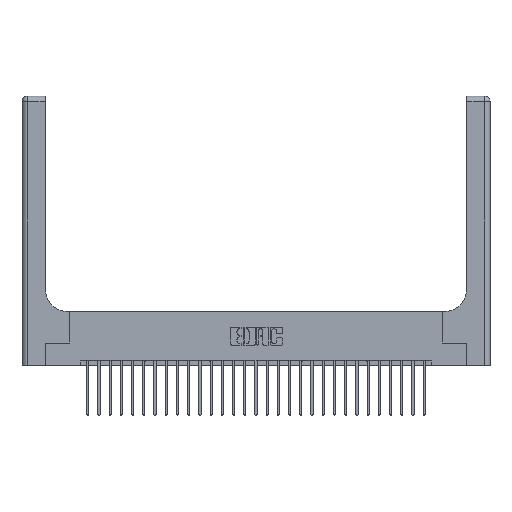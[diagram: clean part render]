
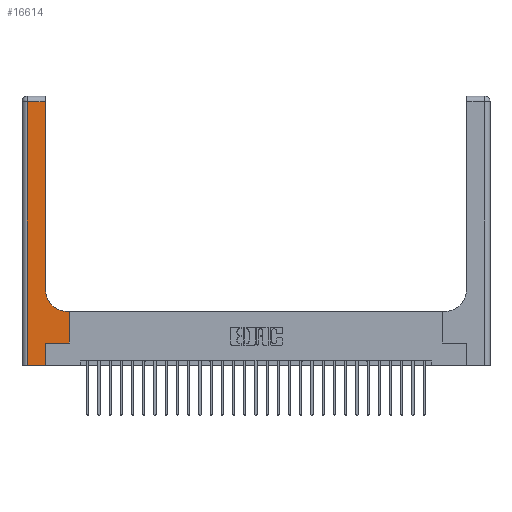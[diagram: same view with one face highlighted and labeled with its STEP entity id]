
A CAD part, top view. The second image highlights one B-rep face of the part: STEP entity #16614.
In plain terms, the highlighted planar face has unit normal (0, 0, 1).
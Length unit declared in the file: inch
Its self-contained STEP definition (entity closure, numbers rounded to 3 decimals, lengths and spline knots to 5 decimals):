
#971 = VERTEX_POINT ( 'NONE', #20135 ) ;
#1554 = DIRECTION ( 'NONE',  ( 0., 0., -1. ) ) ;
#1675 = CARTESIAN_POINT ( 'NONE',  ( 0.06, 0., 0.37 ) ) ;
#1755 = EDGE_CURVE ( 'NONE', #26355, #6353, #17251, .T. ) ;
#1874 = AXIS2_PLACEMENT_3D ( 'NONE', #26475, #1554, #7898 ) ;
#1891 = CARTESIAN_POINT ( 'NONE',  ( 0., 2.94, 0.37 ) ) ;
#2006 = AXIS2_PLACEMENT_3D ( 'NONE', #8430, #20499, #18570 ) ;
#2599 = VERTEX_POINT ( 'NONE', #3505 ) ;
#3308 = VECTOR ( 'NONE', #17036, 39.37008 ) ;
#3505 = CARTESIAN_POINT ( 'NONE',  ( 0.26, 2.94, 0.37 ) ) ;
#4293 = EDGE_CURVE ( 'NONE', #17906, #971, #13842, .T. ) ;
#4550 = CARTESIAN_POINT ( 'NONE',  ( 0.06, 2.94, 0.37 ) ) ;
#6353 = VERTEX_POINT ( 'NONE', #23645 ) ;
#7100 = LINE ( 'NONE', #15888, #16823 ) ;
#7628 = VERTEX_POINT ( 'NONE', #26012 ) ;
#7898 = DIRECTION ( 'NONE',  ( 1., 0., 0. ) ) ;
#8225 = DIRECTION ( 'NONE',  ( -1., 0., 0. ) ) ;
#8430 = CARTESIAN_POINT ( 'NONE',  ( 0., 3., 0.37 ) ) ;
#8504 = ORIENTED_EDGE ( 'NONE', *, *, #1755, .T. ) ;
#9258 = LINE ( 'NONE', #1891, #19678 ) ;
#9851 = CARTESIAN_POINT ( 'NONE',  ( 0.528, 0.25, 0.37 ) ) ;
#10136 = LINE ( 'NONE', #21403, #3308 ) ;
#10142 = ORIENTED_EDGE ( 'NONE', *, *, #13453, .T. ) ;
#11033 = ORIENTED_EDGE ( 'NONE', *, *, #4293, .T. ) ;
#11135 = CARTESIAN_POINT ( 'NONE',  ( 0.528, 0.25, 0.37 ) ) ;
#11795 = ORIENTED_EDGE ( 'NONE', *, *, #24384, .T. ) ;
#12333 = DIRECTION ( 'NONE',  ( 0., -1., 0. ) ) ;
#12612 = EDGE_CURVE ( 'NONE', #7628, #24047, #19291, .T. ) ;
#13453 = EDGE_CURVE ( 'NONE', #6353, #17906, #10136, .T. ) ;
#13520 = ORIENTED_EDGE ( 'NONE', *, *, #19996, .T. ) ;
#13842 = CIRCLE ( 'NONE', #1874, 0.25 ) ;
#14667 = EDGE_CURVE ( 'NONE', #24047, #26355, #23497, .T. ) ;
#14986 = EDGE_CURVE ( 'NONE', #22394, #24453, #15347, .T. ) ;
#15347 = LINE ( 'NONE', #22702, #15992 ) ;
#15888 = CARTESIAN_POINT ( 'NONE',  ( 0.26, 3., 0.37 ) ) ;
#15940 = VECTOR ( 'NONE', #18199, 39.37008 ) ;
#15992 = VECTOR ( 'NONE', #12333, 39.37008 ) ;
#16246 = LINE ( 'NONE', #22407, #26625 ) ;
#16609 = CARTESIAN_POINT ( 'NONE',  ( 0.265, 0., 0.37 ) ) ;
#16614 = ADVANCED_FACE ( 'NONE', ( #19163 ), #22942, .F. ) ;
#16823 = VECTOR ( 'NONE', #17964, 39.37008 ) ;
#17036 = DIRECTION ( 'NONE',  ( -1., 0., 0. ) ) ;
#17251 = LINE ( 'NONE', #9851, #15940 ) ;
#17541 = ORIENTED_EDGE ( 'NONE', *, *, #14986, .T. ) ;
#17906 = VERTEX_POINT ( 'NONE', #18569 ) ;
#17960 = VECTOR ( 'NONE', #18392, 39.37008 ) ;
#17964 = DIRECTION ( 'NONE',  ( 0., 1., 0. ) ) ;
#18199 = DIRECTION ( 'NONE',  ( 0., 1., 0. ) ) ;
#18255 = EDGE_CURVE ( 'NONE', #971, #2599, #7100, .T. ) ;
#18392 = DIRECTION ( 'NONE',  ( 1., 0., 0. ) ) ;
#18569 = CARTESIAN_POINT ( 'NONE',  ( 0.51, 0.6, 0.37 ) ) ;
#18570 = DIRECTION ( 'NONE',  ( -1., 0., 0. ) ) ;
#18850 = ORIENTED_EDGE ( 'NONE', *, *, #14667, .T. ) ;
#19163 = FACE_OUTER_BOUND ( 'NONE', #26632, .T. ) ;
#19291 = LINE ( 'NONE', #16609, #23195 ) ;
#19678 = VECTOR ( 'NONE', #8225, 39.37008 ) ;
#19996 = EDGE_CURVE ( 'NONE', #2599, #22394, #9258, .T. ) ;
#20083 = ORIENTED_EDGE ( 'NONE', *, *, #18255, .T. ) ;
#20135 = CARTESIAN_POINT ( 'NONE',  ( 0.26, 0.85, 0.37 ) ) ;
#20499 = DIRECTION ( 'NONE',  ( 0., 0., -1. ) ) ;
#21375 = CARTESIAN_POINT ( 'NONE',  ( 0.265, 0.25, 0.37 ) ) ;
#21403 = CARTESIAN_POINT ( 'NONE',  ( 0.26, 0.6, 0.37 ) ) ;
#22394 = VERTEX_POINT ( 'NONE', #4550 ) ;
#22407 = CARTESIAN_POINT ( 'NONE',  ( 0., 0., 0.37 ) ) ;
#22494 = ORIENTED_EDGE ( 'NONE', *, *, #12612, .T. ) ;
#22702 = CARTESIAN_POINT ( 'NONE',  ( 0.06, 3., 0.37 ) ) ;
#22942 = PLANE ( 'NONE',  #2006 ) ;
#23195 = VECTOR ( 'NONE', #26857, 39.37008 ) ;
#23497 = LINE ( 'NONE', #24560, #17960 ) ;
#23645 = CARTESIAN_POINT ( 'NONE',  ( 0.528, 0.6, 0.37 ) ) ;
#24047 = VERTEX_POINT ( 'NONE', #21375 ) ;
#24384 = EDGE_CURVE ( 'NONE', #24453, #7628, #16246, .T. ) ;
#24453 = VERTEX_POINT ( 'NONE', #1675 ) ;
#24560 = CARTESIAN_POINT ( 'NONE',  ( 0.265, 0.25, 0.37 ) ) ;
#24581 = DIRECTION ( 'NONE',  ( 1., 0., 0. ) ) ;
#26012 = CARTESIAN_POINT ( 'NONE',  ( 0.265, 0., 0.37 ) ) ;
#26355 = VERTEX_POINT ( 'NONE', #11135 ) ;
#26475 = CARTESIAN_POINT ( 'NONE',  ( 0.51, 0.85, 0.37 ) ) ;
#26625 = VECTOR ( 'NONE', #24581, 39.37008 ) ;
#26632 = EDGE_LOOP ( 'NONE', ( #20083, #13520, #17541, #11795, #22494, #18850, #8504, #10142, #11033 ) ) ;
#26857 = DIRECTION ( 'NONE',  ( 0., 1., 0. ) ) ;
